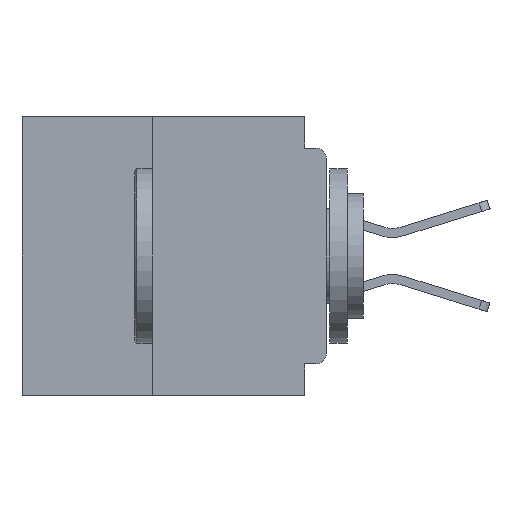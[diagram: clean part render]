
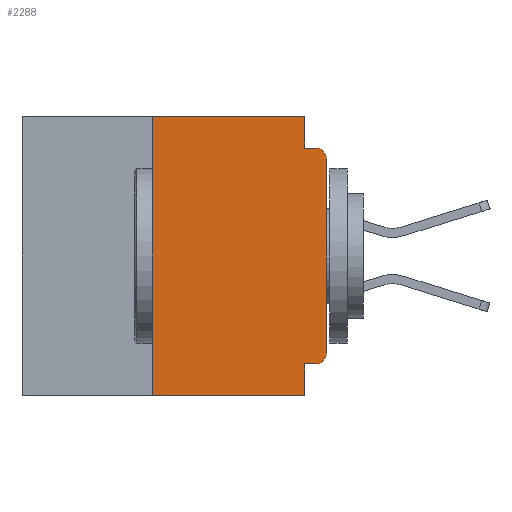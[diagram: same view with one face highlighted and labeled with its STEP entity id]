
A CAD part, left-side view. The second image highlights one B-rep face of the part: STEP entity #2288.
In plain terms, the highlighted planar face has unit normal (-1, 0, 0).
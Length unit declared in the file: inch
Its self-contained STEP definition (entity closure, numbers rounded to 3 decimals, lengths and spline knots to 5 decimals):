
#124 = CARTESIAN_POINT ( 'NONE',  ( 0., 0.031, 0. ) ) ;
#706 = VECTOR ( 'NONE', #20939, 39.37008 ) ;
#1061 = VERTEX_POINT ( 'NONE', #10033 ) ;
#1136 = CARTESIAN_POINT ( 'NONE',  ( 0., 0., 0. ) ) ;
#1528 = EDGE_CURVE ( 'NONE', #29743, #1061, #18474, .T. ) ;
#1784 = LINE ( 'NONE', #124, #706 ) ;
#2288 = ADVANCED_FACE ( 'NONE', ( #7548 ), #17426, .F. ) ;
#2424 = ORIENTED_EDGE ( 'NONE', *, *, #1528, .T. ) ;
#2604 = VECTOR ( 'NONE', #24377, 39.37008 ) ;
#2905 = ORIENTED_EDGE ( 'NONE', *, *, #39118, .F. ) ;
#4042 = CARTESIAN_POINT ( 'NONE',  ( 0., 0.031, -0.4 ) ) ;
#4351 = VERTEX_POINT ( 'NONE', #14707 ) ;
#4421 = VECTOR ( 'NONE', #43005, 39.37008 ) ;
#6013 = LINE ( 'NONE', #33931, #23346 ) ;
#6558 = DIRECTION ( 'NONE',  ( 0., 0., -1. ) ) ;
#6656 = ORIENTED_EDGE ( 'NONE', *, *, #34300, .T. ) ;
#7116 = CARTESIAN_POINT ( 'NONE',  ( 0., 0.25, -0.4 ) ) ;
#7548 = FACE_OUTER_BOUND ( 'NONE', #38005, .T. ) ;
#8084 = DIRECTION ( 'NONE',  ( 0., 0., 1. ) ) ;
#9727 = CARTESIAN_POINT ( 'NONE',  ( 0., 0.25, 0. ) ) ;
#10032 = CARTESIAN_POINT ( 'NONE',  ( 0., 0.031, -0.4 ) ) ;
#10033 = CARTESIAN_POINT ( 'NONE',  ( 0., 0., -0.34 ) ) ;
#11033 = ORIENTED_EDGE ( 'NONE', *, *, #11267, .F. ) ;
#11267 = EDGE_CURVE ( 'NONE', #28142, #22920, #12743, .T. ) ;
#12460 = EDGE_CURVE ( 'NONE', #38193, #22203, #1784, .T. ) ;
#12743 = LINE ( 'NONE', #10032, #29959 ) ;
#13112 = ORIENTED_EDGE ( 'NONE', *, *, #38924, .F. ) ;
#13808 = LINE ( 'NONE', #18412, #43269 ) ;
#14707 = CARTESIAN_POINT ( 'NONE',  ( 0., 0., -0.06 ) ) ;
#17120 = DIRECTION ( 'NONE',  ( 0., -1., 0. ) ) ;
#17426 = PLANE ( 'NONE',  #25813 ) ;
#17987 = CARTESIAN_POINT ( 'NONE',  ( 0., 0.015, -0.045 ) ) ;
#18412 = CARTESIAN_POINT ( 'NONE',  ( 0., 0.437, 0. ) ) ;
#18474 = CIRCLE ( 'NONE', #36954, 0.015 ) ;
#19039 = ORIENTED_EDGE ( 'NONE', *, *, #40406, .T. ) ;
#20223 = CARTESIAN_POINT ( 'NONE',  ( 0., 0.015, -0.34 ) ) ;
#20355 = CARTESIAN_POINT ( 'NONE',  ( 0., 0.015, -0.06 ) ) ;
#20543 = CARTESIAN_POINT ( 'NONE',  ( 0., 0.437, -0.4 ) ) ;
#20939 = DIRECTION ( 'NONE',  ( 0., 0., -1. ) ) ;
#21543 = VERTEX_POINT ( 'NONE', #35928 ) ;
#21696 = CARTESIAN_POINT ( 'NONE',  ( 0., 0.031, 0. ) ) ;
#22100 = VECTOR ( 'NONE', #8084, 39.37008 ) ;
#22203 = VERTEX_POINT ( 'NONE', #22370 ) ;
#22370 = CARTESIAN_POINT ( 'NONE',  ( 0., 0.031, -0.045 ) ) ;
#22880 = ORIENTED_EDGE ( 'NONE', *, *, #40885, .F. ) ;
#22920 = VERTEX_POINT ( 'NONE', #4042 ) ;
#23346 = VECTOR ( 'NONE', #40766, 39.37008 ) ;
#23611 = VECTOR ( 'NONE', #17120, 39.37008 ) ;
#23886 = DIRECTION ( 'NONE',  ( 0., 0., -1. ) ) ;
#23910 = LINE ( 'NONE', #25835, #4421 ) ;
#24377 = DIRECTION ( 'NONE',  ( 0., 0., 1. ) ) ;
#25813 = AXIS2_PLACEMENT_3D ( 'NONE', #41694, #41655, #41512 ) ;
#25835 = CARTESIAN_POINT ( 'NONE',  ( 0., 0., -0.045 ) ) ;
#26024 = CARTESIAN_POINT ( 'NONE',  ( 0., 0.015, -0.355 ) ) ;
#26231 = AXIS2_PLACEMENT_3D ( 'NONE', #20355, #44272, #23886 ) ;
#27872 = EDGE_CURVE ( 'NONE', #4351, #28058, #28358, .T. ) ;
#28058 = VERTEX_POINT ( 'NONE', #17987 ) ;
#28142 = VERTEX_POINT ( 'NONE', #35369 ) ;
#28358 = CIRCLE ( 'NONE', #26231, 0.015 ) ;
#29564 = EDGE_CURVE ( 'NONE', #42556, #38193, #13808, .T. ) ;
#29743 = VERTEX_POINT ( 'NONE', #26024 ) ;
#29959 = VECTOR ( 'NONE', #6558, 39.37008 ) ;
#30325 = ORIENTED_EDGE ( 'NONE', *, *, #27872, .T. ) ;
#30722 = DIRECTION ( 'NONE',  ( 0., 0., -1. ) ) ;
#30812 = DIRECTION ( 'NONE',  ( -1., 0., 0. ) ) ;
#31261 = LINE ( 'NONE', #1136, #22100 ) ;
#33931 = CARTESIAN_POINT ( 'NONE',  ( 0., 0., -0.355 ) ) ;
#34099 = ORIENTED_EDGE ( 'NONE', *, *, #12460, .F. ) ;
#34300 = EDGE_CURVE ( 'NONE', #21543, #22920, #41751, .T. ) ;
#35369 = CARTESIAN_POINT ( 'NONE',  ( 0., 0.031, -0.355 ) ) ;
#35928 = CARTESIAN_POINT ( 'NONE',  ( 0., 0.25, -0.4 ) ) ;
#36793 = ORIENTED_EDGE ( 'NONE', *, *, #29564, .F. ) ;
#36954 = AXIS2_PLACEMENT_3D ( 'NONE', #20223, #30812, #30722 ) ;
#38005 = EDGE_LOOP ( 'NONE', ( #19039, #30325, #13112, #34099, #36793, #22880, #6656, #11033, #2905, #2424 ) ) ;
#38193 = VERTEX_POINT ( 'NONE', #21696 ) ;
#38924 = EDGE_CURVE ( 'NONE', #22203, #28058, #23910, .T. ) ;
#39118 = EDGE_CURVE ( 'NONE', #29743, #28142, #6013, .T. ) ;
#40276 = LINE ( 'NONE', #7116, #2604 ) ;
#40406 = EDGE_CURVE ( 'NONE', #1061, #4351, #31261, .T. ) ;
#40766 = DIRECTION ( 'NONE',  ( 0., 1., 0. ) ) ;
#40885 = EDGE_CURVE ( 'NONE', #21543, #42556, #40276, .T. ) ;
#41512 = DIRECTION ( 'NONE',  ( 0., 0., -1. ) ) ;
#41655 = DIRECTION ( 'NONE',  ( 1., 0., 0. ) ) ;
#41694 = CARTESIAN_POINT ( 'NONE',  ( 0., 0.437, 0. ) ) ;
#41751 = LINE ( 'NONE', #20543, #23611 ) ;
#42317 = DIRECTION ( 'NONE',  ( 0., -1., 0. ) ) ;
#42556 = VERTEX_POINT ( 'NONE', #9727 ) ;
#43005 = DIRECTION ( 'NONE',  ( 0., -1., 0. ) ) ;
#43269 = VECTOR ( 'NONE', #42317, 39.37008 ) ;
#44272 = DIRECTION ( 'NONE',  ( -1., 0., 0. ) ) ;
